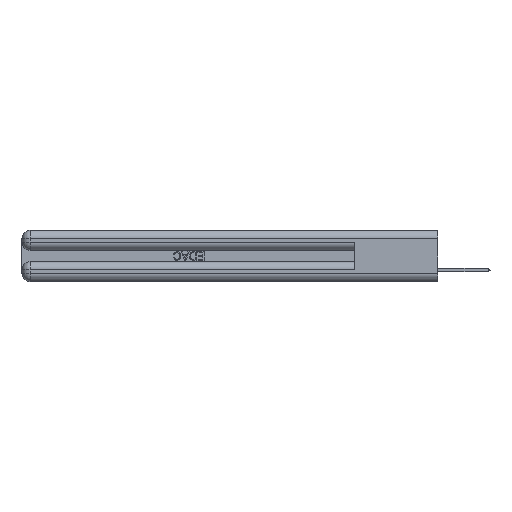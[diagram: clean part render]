
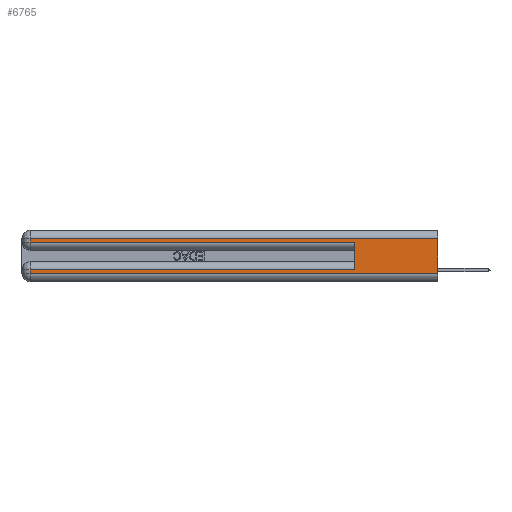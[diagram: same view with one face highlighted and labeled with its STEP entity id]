
A CAD part, left-side view. The second image highlights one B-rep face of the part: STEP entity #6765.
In plain terms, the highlighted planar face has unit normal (-1, 0, 0).
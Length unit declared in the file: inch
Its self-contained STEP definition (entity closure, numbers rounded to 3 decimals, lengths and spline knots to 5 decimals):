
#822 = VECTOR ( 'NONE', #14028, 39.37008 ) ;
#1816 = LINE ( 'NONE', #38495, #47910 ) ;
#5993 = ORIENTED_EDGE ( 'NONE', *, *, #47434, .T. ) ;
#6670 = CARTESIAN_POINT ( 'NONE',  ( 0., 2.94, 0.31 ) ) ;
#6765 = ADVANCED_FACE ( 'NONE', ( #22756 ), #36887, .F. ) ;
#7246 = EDGE_CURVE ( 'NONE', #21609, #28106, #32332, .T. ) ;
#7345 = LINE ( 'NONE', #18099, #822 ) ;
#7856 = CARTESIAN_POINT ( 'NONE',  ( 0., 0., 0.37 ) ) ;
#8055 = VECTOR ( 'NONE', #22668, 39.37008 ) ;
#10174 = CARTESIAN_POINT ( 'NONE',  ( 0., 2.94, 0.37 ) ) ;
#10216 = LINE ( 'NONE', #28645, #19774 ) ;
#10669 = EDGE_CURVE ( 'NONE', #36132, #31192, #10216, .T. ) ;
#13180 = EDGE_CURVE ( 'NONE', #31192, #28106, #14500, .T. ) ;
#13871 = VERTEX_POINT ( 'NONE', #35428 ) ;
#14028 = DIRECTION ( 'NONE',  ( 0., 1., 0. ) ) ;
#14111 = EDGE_CURVE ( 'NONE', #42983, #25670, #48959, .T. ) ;
#14500 = LINE ( 'NONE', #50961, #47101 ) ;
#16309 = DIRECTION ( 'NONE',  ( 0., 0., -1. ) ) ;
#17291 = DIRECTION ( 'NONE',  ( 0., -1., 0. ) ) ;
#17867 = ORIENTED_EDGE ( 'NONE', *, *, #7246, .F. ) ;
#18099 = CARTESIAN_POINT ( 'NONE',  ( 0., 0., 0.085 ) ) ;
#18585 = CARTESIAN_POINT ( 'NONE',  ( 0., 0., 0.06 ) ) ;
#19774 = VECTOR ( 'NONE', #24825, 39.37008 ) ;
#21556 = LINE ( 'NONE', #7856, #26794 ) ;
#21609 = VERTEX_POINT ( 'NONE', #49081 ) ;
#22202 = CARTESIAN_POINT ( 'NONE',  ( 0., 0., 0.31 ) ) ;
#22242 = CARTESIAN_POINT ( 'NONE',  ( 0., 0.6, 0.145 ) ) ;
#22449 = DIRECTION ( 'NONE',  ( 0., 0., 1. ) ) ;
#22668 = DIRECTION ( 'NONE',  ( 0., 0., -1. ) ) ;
#22756 = FACE_OUTER_BOUND ( 'NONE', #25675, .T. ) ;
#24059 = EDGE_CURVE ( 'NONE', #13871, #27634, #21556, .T. ) ;
#24825 = DIRECTION ( 'NONE',  ( 0., 0., -1. ) ) ;
#25670 = VERTEX_POINT ( 'NONE', #40186 ) ;
#25675 = EDGE_LOOP ( 'NONE', ( #46321, #32725, #30190, #37096, #17867, #5993, #41923, #44688 ) ) ;
#26376 = DIRECTION ( 'NONE',  ( 0., 1., 0. ) ) ;
#26794 = VECTOR ( 'NONE', #40170, 39.37008 ) ;
#26964 = EDGE_CURVE ( 'NONE', #13871, #36132, #37882, .T. ) ;
#27634 = VERTEX_POINT ( 'NONE', #18585 ) ;
#28106 = VERTEX_POINT ( 'NONE', #41636 ) ;
#28645 = CARTESIAN_POINT ( 'NONE',  ( 0., 2.94, 0.37 ) ) ;
#30190 = ORIENTED_EDGE ( 'NONE', *, *, #10669, .T. ) ;
#31192 = VERTEX_POINT ( 'NONE', #51562 ) ;
#32332 = LINE ( 'NONE', #22242, #37361 ) ;
#32725 = ORIENTED_EDGE ( 'NONE', *, *, #26964, .T. ) ;
#35428 = CARTESIAN_POINT ( 'NONE',  ( 0., 0., 0.31 ) ) ;
#35729 = AXIS2_PLACEMENT_3D ( 'NONE', #41135, #49656, #16309 ) ;
#35997 = EDGE_CURVE ( 'NONE', #25670, #27634, #1816, .T. ) ;
#36132 = VERTEX_POINT ( 'NONE', #6670 ) ;
#36887 = PLANE ( 'NONE',  #35729 ) ;
#37096 = ORIENTED_EDGE ( 'NONE', *, *, #13180, .T. ) ;
#37361 = VECTOR ( 'NONE', #22449, 39.37008 ) ;
#37882 = LINE ( 'NONE', #22202, #51309 ) ;
#38495 = CARTESIAN_POINT ( 'NONE',  ( 0., 0., 0.06 ) ) ;
#40170 = DIRECTION ( 'NONE',  ( 0., 0., -1. ) ) ;
#40186 = CARTESIAN_POINT ( 'NONE',  ( 0., 2.94, 0.06 ) ) ;
#41135 = CARTESIAN_POINT ( 'NONE',  ( 0., 0., 0.37 ) ) ;
#41294 = CARTESIAN_POINT ( 'NONE',  ( 0., 2.94, 0.085 ) ) ;
#41636 = CARTESIAN_POINT ( 'NONE',  ( 0., 0.6, 0.285 ) ) ;
#41923 = ORIENTED_EDGE ( 'NONE', *, *, #14111, .T. ) ;
#42983 = VERTEX_POINT ( 'NONE', #41294 ) ;
#44688 = ORIENTED_EDGE ( 'NONE', *, *, #35997, .T. ) ;
#46321 = ORIENTED_EDGE ( 'NONE', *, *, #24059, .F. ) ;
#46668 = DIRECTION ( 'NONE',  ( 0., -1., 0. ) ) ;
#47101 = VECTOR ( 'NONE', #46668, 39.37008 ) ;
#47434 = EDGE_CURVE ( 'NONE', #21609, #42983, #7345, .T. ) ;
#47910 = VECTOR ( 'NONE', #17291, 39.37008 ) ;
#48959 = LINE ( 'NONE', #10174, #8055 ) ;
#49081 = CARTESIAN_POINT ( 'NONE',  ( 0., 0.6, 0.085 ) ) ;
#49656 = DIRECTION ( 'NONE',  ( 1., 0., 0. ) ) ;
#50961 = CARTESIAN_POINT ( 'NONE',  ( 0., 0., 0.285 ) ) ;
#51309 = VECTOR ( 'NONE', #26376, 39.37008 ) ;
#51562 = CARTESIAN_POINT ( 'NONE',  ( 0., 2.94, 0.285 ) ) ;
